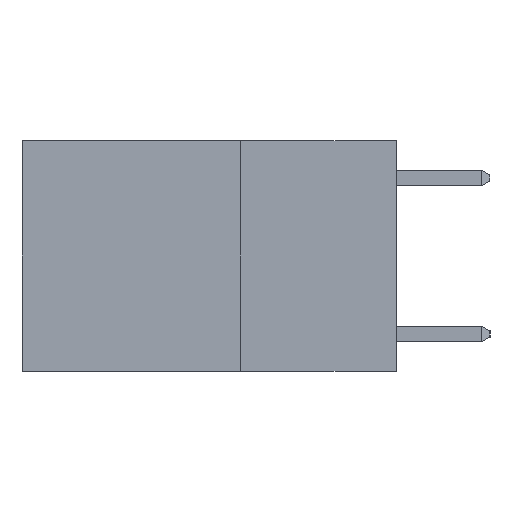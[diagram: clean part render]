
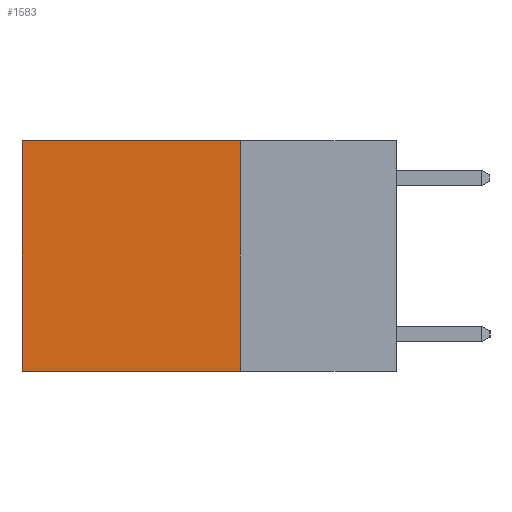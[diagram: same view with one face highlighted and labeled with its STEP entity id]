
A CAD part, left-side view. The second image highlights one B-rep face of the part: STEP entity #1583.
In plain terms, the highlighted planar face has unit normal (-1, 0, 0).
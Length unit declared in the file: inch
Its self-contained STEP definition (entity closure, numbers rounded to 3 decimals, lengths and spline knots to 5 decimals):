
#44 = DIRECTION ( 'NONE',  ( 0., 0., -1. ) ) ;
#170 = LINE ( 'NONE', #9583, #3990 ) ;
#251 = LINE ( 'NONE', #9631, #8348 ) ;
#397 = DIRECTION ( 'NONE',  ( 0., 1., 0. ) ) ;
#445 = VERTEX_POINT ( 'NONE', #3360 ) ;
#888 = VERTEX_POINT ( 'NONE', #9466 ) ;
#1104 = LINE ( 'NONE', #1165, #8967 ) ;
#1165 = CARTESIAN_POINT ( 'NONE',  ( 0.2625, 0.25, -0.37 ) ) ;
#1268 = ORIENTED_EDGE ( 'NONE', *, *, #5686, .T. ) ;
#1583 = ADVANCED_FACE ( 'NONE', ( #7240 ), #6417, .F. ) ;
#1898 = CARTESIAN_POINT ( 'NONE',  ( 0.2625, 0.25, 0. ) ) ;
#2197 = VERTEX_POINT ( 'NONE', #3595 ) ;
#2394 = EDGE_CURVE ( 'NONE', #445, #888, #9454, .T. ) ;
#2439 = AXIS2_PLACEMENT_3D ( 'NONE', #1898, #7988, #3434 ) ;
#3168 = VECTOR ( 'NONE', #44, 39.37008 ) ;
#3360 = CARTESIAN_POINT ( 'NONE',  ( 0.2625, 0.6, 0. ) ) ;
#3434 = DIRECTION ( 'NONE',  ( 0., 0., -1. ) ) ;
#3444 = EDGE_CURVE ( 'NONE', #9012, #2197, #170, .T. ) ;
#3595 = CARTESIAN_POINT ( 'NONE',  ( 0.2625, 0.25, -0.37 ) ) ;
#3844 = CARTESIAN_POINT ( 'NONE',  ( 0.2625, 0.6, 0. ) ) ;
#3990 = VECTOR ( 'NONE', #4299, 39.37008 ) ;
#4299 = DIRECTION ( 'NONE',  ( 0., 0., -1. ) ) ;
#5064 = DIRECTION ( 'NONE',  ( 0., 1., 0. ) ) ;
#5231 = EDGE_LOOP ( 'NONE', ( #5924, #8255, #9578, #1268 ) ) ;
#5686 = EDGE_CURVE ( 'NONE', #9012, #445, #251, .T. ) ;
#5924 = ORIENTED_EDGE ( 'NONE', *, *, #2394, .T. ) ;
#6417 = PLANE ( 'NONE',  #2439 ) ;
#6841 = EDGE_CURVE ( 'NONE', #2197, #888, #1104, .T. ) ;
#7240 = FACE_OUTER_BOUND ( 'NONE', #5231, .T. ) ;
#7703 = CARTESIAN_POINT ( 'NONE',  ( 0.2625, 0.25, 0. ) ) ;
#7988 = DIRECTION ( 'NONE',  ( 1., 0., 0. ) ) ;
#8255 = ORIENTED_EDGE ( 'NONE', *, *, #6841, .F. ) ;
#8348 = VECTOR ( 'NONE', #5064, 39.37008 ) ;
#8967 = VECTOR ( 'NONE', #397, 39.37008 ) ;
#9012 = VERTEX_POINT ( 'NONE', #7703 ) ;
#9454 = LINE ( 'NONE', #3844, #3168 ) ;
#9466 = CARTESIAN_POINT ( 'NONE',  ( 0.2625, 0.6, -0.37 ) ) ;
#9578 = ORIENTED_EDGE ( 'NONE', *, *, #3444, .F. ) ;
#9583 = CARTESIAN_POINT ( 'NONE',  ( 0.2625, 0.25, 0. ) ) ;
#9631 = CARTESIAN_POINT ( 'NONE',  ( 0.2625, 0.25, 0. ) ) ;
